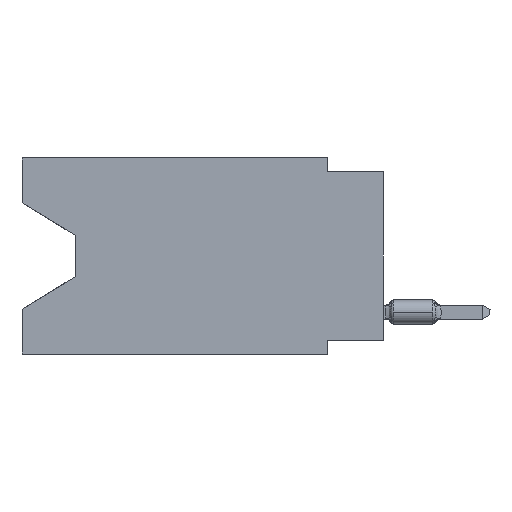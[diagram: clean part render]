
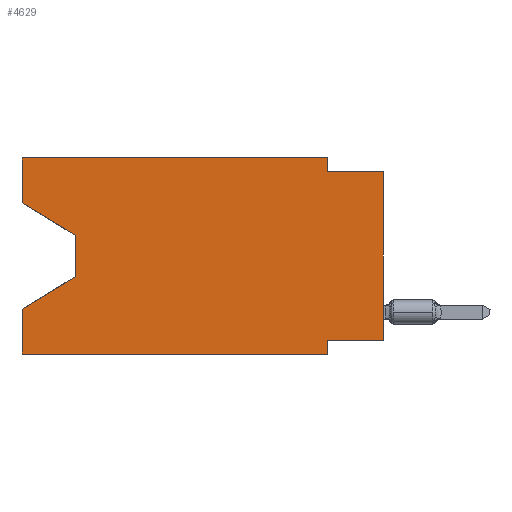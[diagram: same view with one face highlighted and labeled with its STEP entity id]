
A CAD part, left-side view. The second image highlights one B-rep face of the part: STEP entity #4629.
In plain terms, the highlighted planar face has unit normal (-1, 0, 0).
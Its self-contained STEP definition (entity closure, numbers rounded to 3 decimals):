
#227 = VERTEX_POINT ( 'NONE', #10880 ) ;
#684 = ORIENTED_EDGE ( 'NONE', *, *, #17927, .T. ) ;
#811 = VECTOR ( 'NONE', #30181, 1000. ) ;
#978 = VERTEX_POINT ( 'NONE', #35853 ) ;
#1111 = LINE ( 'NONE', #7212, #34791 ) ;
#1252 = LINE ( 'NONE', #35756, #811 ) ;
#1540 = LINE ( 'NONE', #12865, #22077 ) ;
#1975 = VECTOR ( 'NONE', #36393, 1000. ) ;
#2358 = CARTESIAN_POINT ( 'NONE',  ( 0., 16.383, -6.852 ) ) ;
#3180 = ORIENTED_EDGE ( 'NONE', *, *, #26705, .F. ) ;
#4111 = FACE_OUTER_BOUND ( 'NONE', #29471, .T. ) ;
#4259 = EDGE_CURVE ( 'NONE', #8279, #33448, #11563, .T. ) ;
#4340 = ORIENTED_EDGE ( 'NONE', *, *, #15892, .F. ) ;
#4629 = ADVANCED_FACE ( 'NONE', ( #4111 ), #7268, .F. ) ;
#4661 = DIRECTION ( 'NONE',  ( 1., 0., 0. ) ) ;
#4688 = CARTESIAN_POINT ( 'NONE',  ( 0., 0., -8.255 ) ) ;
#5647 = EDGE_CURVE ( 'NONE', #227, #21904, #1111, .T. ) ;
#5829 = ORIENTED_EDGE ( 'NONE', *, *, #16747, .T. ) ;
#5918 = VECTOR ( 'NONE', #32815, 1000. ) ;
#7164 = ORIENTED_EDGE ( 'NONE', *, *, #19508, .T. ) ;
#7212 = CARTESIAN_POINT ( 'NONE',  ( 0., 13.97, -5.385 ) ) ;
#7268 = PLANE ( 'NONE',  #25252 ) ;
#8279 = VERTEX_POINT ( 'NONE', #8668 ) ;
#8421 = LINE ( 'NONE', #16098, #14568 ) ;
#8668 = CARTESIAN_POINT ( 'NONE',  ( 0., 2.54, -8.255 ) ) ;
#8933 = EDGE_CURVE ( 'NONE', #35421, #32535, #13241, .T. ) ;
#9405 = DIRECTION ( 'NONE',  ( 0., 0., -1. ) ) ;
#9762 = ORIENTED_EDGE ( 'NONE', *, *, #27551, .F. ) ;
#10615 = DIRECTION ( 'NONE',  ( 0., 0., 1. ) ) ;
#10826 = CARTESIAN_POINT ( 'NONE',  ( 0., 2.54, -8.89 ) ) ;
#10880 = CARTESIAN_POINT ( 'NONE',  ( 0., 13.97, -5.385 ) ) ;
#11157 = CARTESIAN_POINT ( 'NONE',  ( 0., 0., -0.635 ) ) ;
#11563 = LINE ( 'NONE', #10826, #33567 ) ;
#12219 = EDGE_CURVE ( 'NONE', #27705, #23756, #13758, .T. ) ;
#12865 = CARTESIAN_POINT ( 'NONE',  ( 0., 16.383, 0. ) ) ;
#13050 = DIRECTION ( 'NONE',  ( 0., -0.855, -0.519 ) ) ;
#13241 = LINE ( 'NONE', #18814, #28122 ) ;
#13519 = LINE ( 'NONE', #27242, #5918 ) ;
#13624 = CARTESIAN_POINT ( 'NONE',  ( 0., 16.383, 0. ) ) ;
#13758 = LINE ( 'NONE', #11157, #1975 ) ;
#14568 = VECTOR ( 'NONE', #22360, 1000. ) ;
#14976 = VERTEX_POINT ( 'NONE', #4688 ) ;
#15107 = CARTESIAN_POINT ( 'NONE',  ( 0., 2.54, 0. ) ) ;
#15410 = VECTOR ( 'NONE', #16104, 1000. ) ;
#15437 = DIRECTION ( 'NONE',  ( 0., 1., 0. ) ) ;
#15526 = CARTESIAN_POINT ( 'NONE',  ( 0., 2.54, 0. ) ) ;
#15892 = EDGE_CURVE ( 'NONE', #35421, #30058, #1540, .T. ) ;
#15982 = CARTESIAN_POINT ( 'NONE',  ( 0., 2.54, -0.635 ) ) ;
#15986 = DIRECTION ( 'NONE',  ( 0., 0., -1. ) ) ;
#16098 = CARTESIAN_POINT ( 'NONE',  ( 0., 0., 0. ) ) ;
#16104 = DIRECTION ( 'NONE',  ( 0., 0., -1. ) ) ;
#16747 = EDGE_CURVE ( 'NONE', #978, #33448, #1252, .T. ) ;
#17927 = EDGE_CURVE ( 'NONE', #32535, #227, #29641, .T. ) ;
#18814 = CARTESIAN_POINT ( 'NONE',  ( 0., 16.383, -2.038 ) ) ;
#19508 = EDGE_CURVE ( 'NONE', #14976, #23756, #8421, .T. ) ;
#19931 = ORIENTED_EDGE ( 'NONE', *, *, #12219, .F. ) ;
#20279 = VECTOR ( 'NONE', #24024, 1000. ) ;
#20304 = CARTESIAN_POINT ( 'NONE',  ( 0., 16.383, 0. ) ) ;
#21148 = DIRECTION ( 'NONE',  ( 0., 0.855, -0.519 ) ) ;
#21185 = CARTESIAN_POINT ( 'NONE',  ( 0., 0., -8.255 ) ) ;
#21904 = VERTEX_POINT ( 'NONE', #2358 ) ;
#22077 = VECTOR ( 'NONE', #10615, 1000. ) ;
#22360 = DIRECTION ( 'NONE',  ( 0., 0., 1. ) ) ;
#22551 = EDGE_CURVE ( 'NONE', #978, #21904, #32368, .T. ) ;
#23363 = VERTEX_POINT ( 'NONE', #15107 ) ;
#23756 = VERTEX_POINT ( 'NONE', #28958 ) ;
#24024 = DIRECTION ( 'NONE',  ( 0., 0., 1. ) ) ;
#24769 = ORIENTED_EDGE ( 'NONE', *, *, #5647, .T. ) ;
#25252 = AXIS2_PLACEMENT_3D ( 'NONE', #32874, #4661, #15986 ) ;
#26705 = EDGE_CURVE ( 'NONE', #30058, #23363, #13519, .T. ) ;
#27242 = CARTESIAN_POINT ( 'NONE',  ( 0., 16.383, 0. ) ) ;
#27551 = EDGE_CURVE ( 'NONE', #14976, #8279, #32496, .T. ) ;
#27705 = VERTEX_POINT ( 'NONE', #15982 ) ;
#27840 = CARTESIAN_POINT ( 'NONE',  ( 0., 13.97, -3.505 ) ) ;
#28122 = VECTOR ( 'NONE', #13050, 1000. ) ;
#28298 = EDGE_CURVE ( 'NONE', #23363, #27705, #32232, .T. ) ;
#28958 = CARTESIAN_POINT ( 'NONE',  ( 0., 0., -0.635 ) ) ;
#29324 = ORIENTED_EDGE ( 'NONE', *, *, #28298, .F. ) ;
#29471 = EDGE_LOOP ( 'NONE', ( #34264, #684, #24769, #33947, #5829, #34909, #9762, #7164, #19931, #29324, #3180, #4340 ) ) ;
#29641 = LINE ( 'NONE', #32445, #15410 ) ;
#30058 = VERTEX_POINT ( 'NONE', #13624 ) ;
#30181 = DIRECTION ( 'NONE',  ( 0., -1., 0. ) ) ;
#30286 = VECTOR ( 'NONE', #15437, 1000. ) ;
#30503 = CARTESIAN_POINT ( 'NONE',  ( 0., 16.383, -2.038 ) ) ;
#32232 = LINE ( 'NONE', #15526, #33884 ) ;
#32368 = LINE ( 'NONE', #20304, #20279 ) ;
#32445 = CARTESIAN_POINT ( 'NONE',  ( 0., 13.97, -3.505 ) ) ;
#32496 = LINE ( 'NONE', #21185, #30286 ) ;
#32535 = VERTEX_POINT ( 'NONE', #27840 ) ;
#32815 = DIRECTION ( 'NONE',  ( 0., -1., 0. ) ) ;
#32874 = CARTESIAN_POINT ( 'NONE',  ( 0., 16.383, 0. ) ) ;
#33448 = VERTEX_POINT ( 'NONE', #35110 ) ;
#33567 = VECTOR ( 'NONE', #34194, 1000. ) ;
#33884 = VECTOR ( 'NONE', #9405, 1000. ) ;
#33947 = ORIENTED_EDGE ( 'NONE', *, *, #22551, .F. ) ;
#34194 = DIRECTION ( 'NONE',  ( 0., 0., -1. ) ) ;
#34264 = ORIENTED_EDGE ( 'NONE', *, *, #8933, .T. ) ;
#34791 = VECTOR ( 'NONE', #21148, 1000. ) ;
#34909 = ORIENTED_EDGE ( 'NONE', *, *, #4259, .F. ) ;
#35110 = CARTESIAN_POINT ( 'NONE',  ( 0., 2.54, -8.89 ) ) ;
#35421 = VERTEX_POINT ( 'NONE', #30503 ) ;
#35756 = CARTESIAN_POINT ( 'NONE',  ( 0., 16.383, -8.89 ) ) ;
#35853 = CARTESIAN_POINT ( 'NONE',  ( 0., 16.383, -8.89 ) ) ;
#36393 = DIRECTION ( 'NONE',  ( 0., -1., 0. ) ) ;
